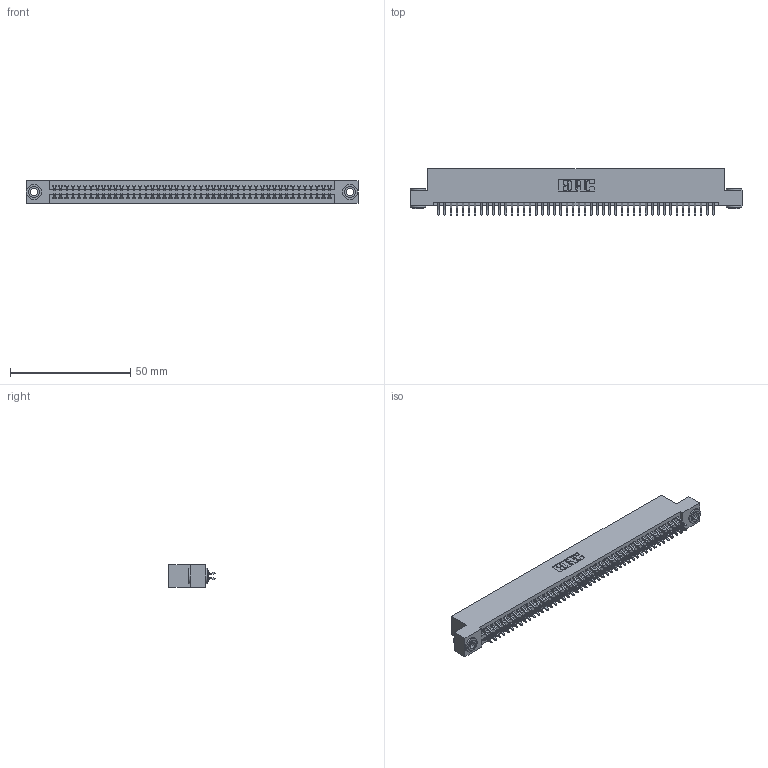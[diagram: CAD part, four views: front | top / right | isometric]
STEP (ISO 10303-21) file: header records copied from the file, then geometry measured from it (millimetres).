
FILE_DESCRIPTION (( 'STEP AP203' ), '1' );
FILE_NAME ('345-092-556-203.STEP', '2018-10-04T22:03:16', ( '' ), ( '' ), 'SwSTEP 2.0', 'SolidWorks 2016', '' );
FILE_SCHEMA (( 'CONFIG_CONTROL_DESIGN' ));
Length unit declared in the file: inch
Products named in the file (4): 345-292-001_556 Tail; 345-250-002_345-250-002-102; 345-092-556-203; 345 Part_Flush Mounting Lugs - 0.156 Dia-TH
Assembly tree (95 placements, depth 2):
  345-092-556-203
    345 Part_Flush Mounting Lugs - 0.156 Dia-TH
    345-292-001_556 Tail  x92
    345-250-002_345-250-002-102  x2
Bounding box: 138.05 x 19.24 x 9.4 mm (x, y, z)
Volume: 13463.1 mm3; surface area: 20102.6 mm2
Topology: 95 solids, 95 shells, 5316 faces, 15781 edges, 10394 vertices
Faces by surface type: plane 3494, cylinder 1814, cone 8
Entity records: 36424 total; most frequent: CARTESIAN_POINT 6091, ORIENTED_EDGE 6006, DIRECTION 5385, EDGE_CURVE 3003, LINE 2655, VECTOR 2655, VERTEX_POINT 1998, AXIS2_PLACEMENT_3D 1365
